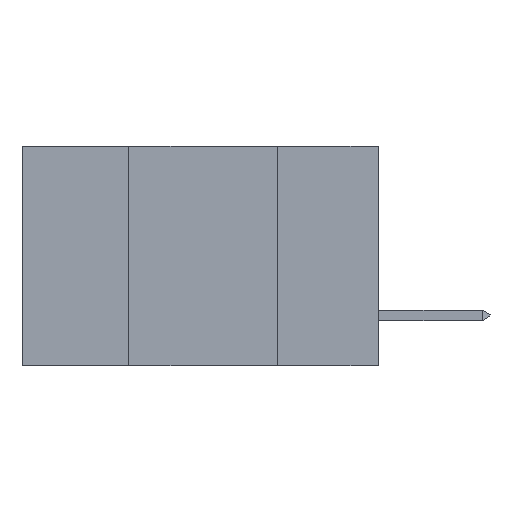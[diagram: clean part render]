
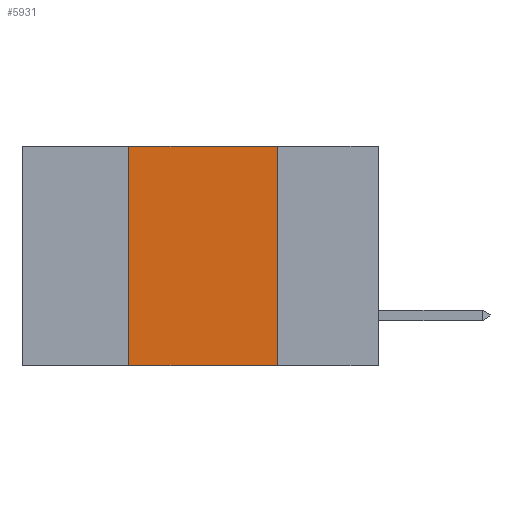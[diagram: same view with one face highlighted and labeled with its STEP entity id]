
A CAD part, left-side view. The second image highlights one B-rep face of the part: STEP entity #5931.
In plain terms, the highlighted planar face has unit normal (-1, 0, 0).
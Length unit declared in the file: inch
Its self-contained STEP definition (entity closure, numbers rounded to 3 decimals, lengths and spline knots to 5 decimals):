
#136 = VERTEX_POINT ( 'NONE', #2406 ) ;
#589 = DIRECTION ( 'NONE',  ( 0., 0., -1. ) ) ;
#644 = EDGE_CURVE ( 'NONE', #9310, #7310, #3805, .T. ) ;
#654 = CARTESIAN_POINT ( 'NONE',  ( 0., 0.6, 0. ) ) ;
#1273 = CARTESIAN_POINT ( 'NONE',  ( 0., 0.17, 0. ) ) ;
#1284 = CARTESIAN_POINT ( 'NONE',  ( 0., 0.6, 0. ) ) ;
#2060 = EDGE_CURVE ( 'NONE', #10356, #136, #5769, .T. ) ;
#2071 = CARTESIAN_POINT ( 'NONE',  ( 0., 0.17, -0.37 ) ) ;
#2406 = CARTESIAN_POINT ( 'NONE',  ( 0., 0.42, 0. ) ) ;
#2416 = VECTOR ( 'NONE', #589, 39.37008 ) ;
#2652 = VECTOR ( 'NONE', #2657, 39.37008 ) ;
#2657 = DIRECTION ( 'NONE',  ( 0., 0., 1. ) ) ;
#2925 = DIRECTION ( 'NONE',  ( 0., -1., 0. ) ) ;
#3268 = FACE_OUTER_BOUND ( 'NONE', #3417, .T. ) ;
#3417 = EDGE_LOOP ( 'NONE', ( #6121, #9114, #10271, #3433 ) ) ;
#3433 = ORIENTED_EDGE ( 'NONE', *, *, #9196, .T. ) ;
#3805 = LINE ( 'NONE', #7017, #2416 ) ;
#4367 = CARTESIAN_POINT ( 'NONE',  ( 0., 0.42, -0.37 ) ) ;
#4420 = EDGE_CURVE ( 'NONE', #136, #9310, #6930, .T. ) ;
#4919 = DIRECTION ( 'NONE',  ( 1., 0., 0. ) ) ;
#5769 = LINE ( 'NONE', #6659, #2652 ) ;
#5931 = ADVANCED_FACE ( 'NONE', ( #3268 ), #6388, .F. ) ;
#6121 = ORIENTED_EDGE ( 'NONE', *, *, #644, .F. ) ;
#6388 = PLANE ( 'NONE',  #7903 ) ;
#6659 = CARTESIAN_POINT ( 'NONE',  ( 0., 0.42, -0.37 ) ) ;
#6930 = LINE ( 'NONE', #1284, #10430 ) ;
#7017 = CARTESIAN_POINT ( 'NONE',  ( 0., 0.17, -0.37 ) ) ;
#7310 = VERTEX_POINT ( 'NONE', #2071 ) ;
#7837 = VECTOR ( 'NONE', #9061, 39.37008 ) ;
#7903 = AXIS2_PLACEMENT_3D ( 'NONE', #654, #4919, #8141 ) ;
#8141 = DIRECTION ( 'NONE',  ( 0., 0., -1. ) ) ;
#9061 = DIRECTION ( 'NONE',  ( 0., -1., 0. ) ) ;
#9114 = ORIENTED_EDGE ( 'NONE', *, *, #4420, .F. ) ;
#9171 = LINE ( 'NONE', #9863, #7837 ) ;
#9196 = EDGE_CURVE ( 'NONE', #10356, #7310, #9171, .T. ) ;
#9310 = VERTEX_POINT ( 'NONE', #1273 ) ;
#9863 = CARTESIAN_POINT ( 'NONE',  ( 0., 0.6, -0.37 ) ) ;
#10271 = ORIENTED_EDGE ( 'NONE', *, *, #2060, .F. ) ;
#10356 = VERTEX_POINT ( 'NONE', #4367 ) ;
#10430 = VECTOR ( 'NONE', #2925, 39.37008 ) ;
